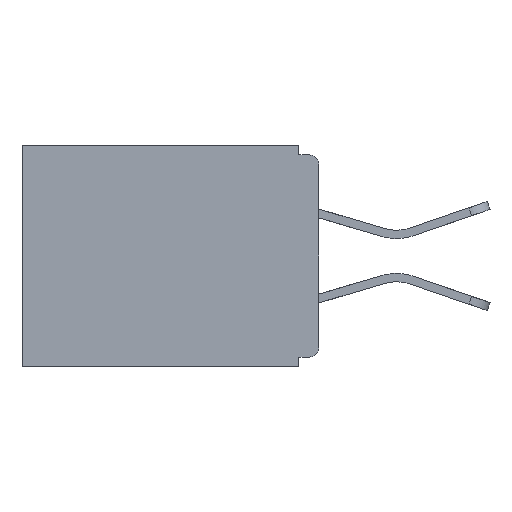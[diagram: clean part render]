
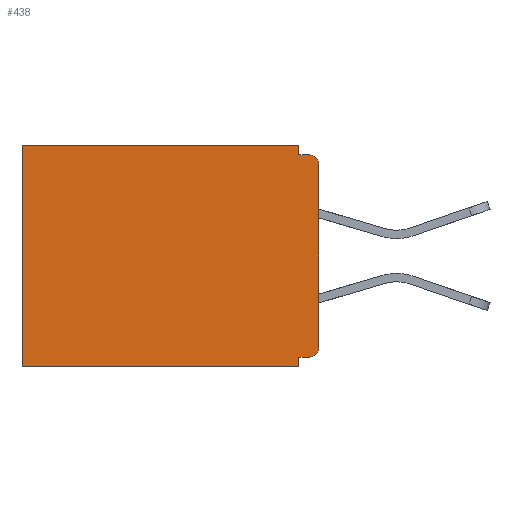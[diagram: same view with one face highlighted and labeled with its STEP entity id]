
A CAD part, left-side view. The second image highlights one B-rep face of the part: STEP entity #438.
In plain terms, the highlighted planar face has unit normal (-1, 0, 0).
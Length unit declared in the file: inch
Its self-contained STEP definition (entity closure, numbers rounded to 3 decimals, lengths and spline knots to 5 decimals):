
#43 = DIRECTION ( 'NONE',  ( 0., 1., 0. ) ) ;
#242 = VERTEX_POINT ( 'NONE', #9440 ) ;
#433 = ORIENTED_EDGE ( 'NONE', *, *, #12672, .T. ) ;
#438 = ADVANCED_FACE ( 'NONE', ( #5545 ), #12823, .F. ) ;
#605 = DIRECTION ( 'NONE',  ( 0., 0., -1. ) ) ;
#833 = CARTESIAN_POINT ( 'NONE',  ( 0.298, 0.46, 0. ) ) ;
#846 = ORIENTED_EDGE ( 'NONE', *, *, #7642, .F. ) ;
#872 = DIRECTION ( 'NONE',  ( 0., 1., 0. ) ) ;
#897 = CARTESIAN_POINT ( 'NONE',  ( 0.298, 0., -0.313 ) ) ;
#926 = CARTESIAN_POINT ( 'NONE',  ( 0.298, 0.031, -0.343 ) ) ;
#995 = DIRECTION ( 'NONE',  ( -1., 0., 0. ) ) ;
#1121 = LINE ( 'NONE', #926, #7605 ) ;
#1403 = CARTESIAN_POINT ( 'NONE',  ( 0.298, 0.031, 0. ) ) ;
#1408 = CIRCLE ( 'NONE', #6053, 0.015 ) ;
#1498 = CARTESIAN_POINT ( 'NONE',  ( 0.298, 0.031, -0.015 ) ) ;
#1679 = DIRECTION ( 'NONE',  ( 0., 0., -1. ) ) ;
#1793 = DIRECTION ( 'NONE',  ( 0., 1., 0. ) ) ;
#1797 = ORIENTED_EDGE ( 'NONE', *, *, #10014, .F. ) ;
#2030 = DIRECTION ( 'NONE',  ( 0., 0., -1. ) ) ;
#2083 = CARTESIAN_POINT ( 'NONE',  ( 0.298, 0., -0.343 ) ) ;
#2389 = VERTEX_POINT ( 'NONE', #833 ) ;
#2533 = LINE ( 'NONE', #3811, #3332 ) ;
#2878 = VERTEX_POINT ( 'NONE', #1403 ) ;
#2937 = DIRECTION ( 'NONE',  ( 0., 0., -1. ) ) ;
#3332 = VECTOR ( 'NONE', #872, 39.37008 ) ;
#3429 = VERTEX_POINT ( 'NONE', #10814 ) ;
#3792 = DIRECTION ( 'NONE',  ( 0., -1., 0. ) ) ;
#3811 = CARTESIAN_POINT ( 'NONE',  ( 0.298, 0., -0.328 ) ) ;
#3822 = VECTOR ( 'NONE', #3792, 39.37008 ) ;
#3833 = EDGE_CURVE ( 'NONE', #9410, #11356, #5961, .T. ) ;
#3907 = CARTESIAN_POINT ( 'NONE',  ( 0.298, 0., -0.03 ) ) ;
#4066 = DIRECTION ( 'NONE',  ( 0., 0., -1. ) ) ;
#4457 = ORIENTED_EDGE ( 'NONE', *, *, #3833, .F. ) ;
#4547 = VECTOR ( 'NONE', #2937, 39.37008 ) ;
#4582 = LINE ( 'NONE', #10050, #8895 ) ;
#4647 = VERTEX_POINT ( 'NONE', #11942 ) ;
#5361 = CARTESIAN_POINT ( 'NONE',  ( 0.298, 0., -0.015 ) ) ;
#5545 = FACE_OUTER_BOUND ( 'NONE', #6439, .T. ) ;
#5692 = DIRECTION ( 'NONE',  ( 1., 0., 0. ) ) ;
#5961 = LINE ( 'NONE', #2083, #13120 ) ;
#6040 = VECTOR ( 'NONE', #605, 39.37008 ) ;
#6053 = AXIS2_PLACEMENT_3D ( 'NONE', #10026, #995, #2030 ) ;
#6420 = EDGE_CURVE ( 'NONE', #2389, #11356, #7287, .T. ) ;
#6439 = EDGE_LOOP ( 'NONE', ( #8554, #8773, #6983, #10946, #9773, #4457, #1797, #10631, #433, #846 ) ) ;
#6732 = EDGE_CURVE ( 'NONE', #2878, #2389, #4582, .T. ) ;
#6983 = ORIENTED_EDGE ( 'NONE', *, *, #11134, .F. ) ;
#7245 = LINE ( 'NONE', #9762, #4547 ) ;
#7287 = LINE ( 'NONE', #12747, #6040 ) ;
#7431 = EDGE_CURVE ( 'NONE', #3429, #242, #2533, .T. ) ;
#7532 = EDGE_CURVE ( 'NONE', #9969, #4647, #10789, .T. ) ;
#7605 = VECTOR ( 'NONE', #13099, 39.37008 ) ;
#7631 = VECTOR ( 'NONE', #4066, 39.37008 ) ;
#7642 = EDGE_CURVE ( 'NONE', #9969, #9896, #7245, .T. ) ;
#7881 = VERTEX_POINT ( 'NONE', #1498 ) ;
#7933 = LINE ( 'NONE', #5361, #3822 ) ;
#8215 = DIRECTION ( 'NONE',  ( 0., 0., -1. ) ) ;
#8554 = ORIENTED_EDGE ( 'NONE', *, *, #7532, .T. ) ;
#8773 = ORIENTED_EDGE ( 'NONE', *, *, #11322, .F. ) ;
#8895 = VECTOR ( 'NONE', #1793, 39.37008 ) ;
#9388 = LINE ( 'NONE', #11267, #7631 ) ;
#9410 = VERTEX_POINT ( 'NONE', #9744 ) ;
#9440 = CARTESIAN_POINT ( 'NONE',  ( 0.298, 0.031, -0.328 ) ) ;
#9744 = CARTESIAN_POINT ( 'NONE',  ( 0.298, 0.031, -0.343 ) ) ;
#9762 = CARTESIAN_POINT ( 'NONE',  ( 0.298, 0., 0. ) ) ;
#9773 = ORIENTED_EDGE ( 'NONE', *, *, #6420, .T. ) ;
#9875 = CARTESIAN_POINT ( 'NONE',  ( 0.298, 0.46, -0.343 ) ) ;
#9896 = VERTEX_POINT ( 'NONE', #897 ) ;
#9969 = VERTEX_POINT ( 'NONE', #3907 ) ;
#10014 = EDGE_CURVE ( 'NONE', #242, #9410, #9388, .T. ) ;
#10026 = CARTESIAN_POINT ( 'NONE',  ( 0.298, 0.015, -0.313 ) ) ;
#10050 = CARTESIAN_POINT ( 'NONE',  ( 0.298, 0., 0. ) ) ;
#10631 = ORIENTED_EDGE ( 'NONE', *, *, #7431, .F. ) ;
#10690 = AXIS2_PLACEMENT_3D ( 'NONE', #13162, #12203, #8215 ) ;
#10789 = CIRCLE ( 'NONE', #10690, 0.015 ) ;
#10814 = CARTESIAN_POINT ( 'NONE',  ( 0.298, 0.015, -0.328 ) ) ;
#10946 = ORIENTED_EDGE ( 'NONE', *, *, #6732, .T. ) ;
#11134 = EDGE_CURVE ( 'NONE', #2878, #7881, #1121, .T. ) ;
#11267 = CARTESIAN_POINT ( 'NONE',  ( 0.298, 0.031, -0.343 ) ) ;
#11322 = EDGE_CURVE ( 'NONE', #7881, #4647, #7933, .T. ) ;
#11356 = VERTEX_POINT ( 'NONE', #9875 ) ;
#11824 = AXIS2_PLACEMENT_3D ( 'NONE', #11846, #5692, #1679 ) ;
#11846 = CARTESIAN_POINT ( 'NONE',  ( 0.298, 0., 0. ) ) ;
#11942 = CARTESIAN_POINT ( 'NONE',  ( 0.298, 0.015, -0.015 ) ) ;
#12203 = DIRECTION ( 'NONE',  ( -1., 0., 0. ) ) ;
#12672 = EDGE_CURVE ( 'NONE', #3429, #9896, #1408, .T. ) ;
#12747 = CARTESIAN_POINT ( 'NONE',  ( 0.298, 0.46, 0. ) ) ;
#12823 = PLANE ( 'NONE',  #11824 ) ;
#13099 = DIRECTION ( 'NONE',  ( 0., 0., -1. ) ) ;
#13120 = VECTOR ( 'NONE', #43, 39.37008 ) ;
#13162 = CARTESIAN_POINT ( 'NONE',  ( 0.298, 0.015, -0.03 ) ) ;
